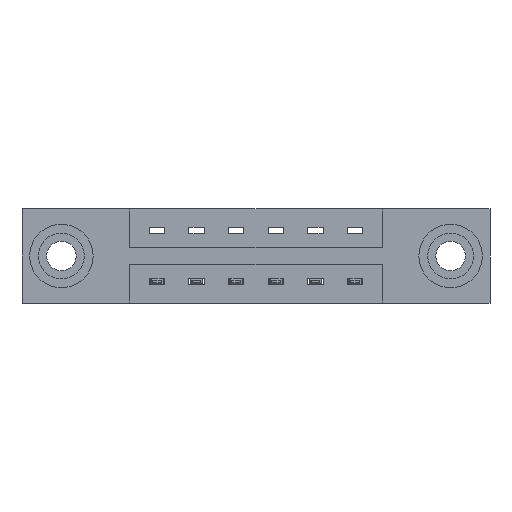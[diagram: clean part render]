
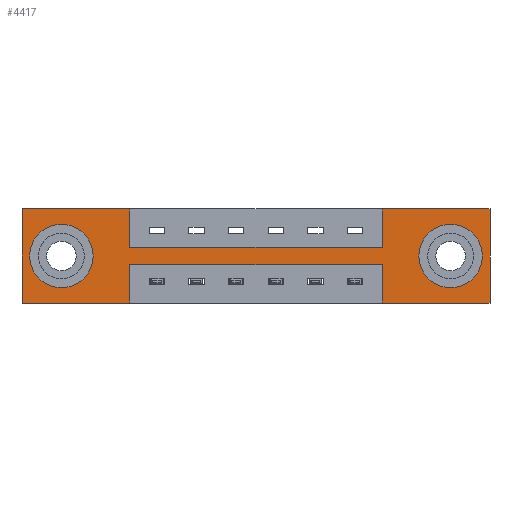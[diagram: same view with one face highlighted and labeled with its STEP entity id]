
A CAD part, front view. The second image highlights one B-rep face of the part: STEP entity #4417.
In plain terms, the highlighted planar face has unit normal (0, -1, 0).
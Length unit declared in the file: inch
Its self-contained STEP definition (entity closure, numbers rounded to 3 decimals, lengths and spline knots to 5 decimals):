
#157 = DIRECTION ( 'NONE',  ( 0., 1., 0. ) ) ;
#269 = LINE ( 'NONE', #6003, #1563 ) ;
#312 = DIRECTION ( 'NONE',  ( 0., 1., 0. ) ) ;
#375 = CARTESIAN_POINT ( 'NONE',  ( 1.842, 0., 0. ) ) ;
#409 = CARTESIAN_POINT ( 'NONE',  ( 0.155, 0., -0.185 ) ) ;
#509 = EDGE_CURVE ( 'NONE', #6867, #2785, #5692, .T. ) ;
#569 = LINE ( 'NONE', #9338, #5206 ) ;
#635 = EDGE_CURVE ( 'NONE', #3390, #4020, #8499, .T. ) ;
#655 = CARTESIAN_POINT ( 'NONE',  ( 1.842, 0., -0.37 ) ) ;
#848 = CARTESIAN_POINT ( 'NONE',  ( 0., 0., 0. ) ) ;
#894 = VERTEX_POINT ( 'NONE', #7296 ) ;
#914 = DIRECTION ( 'NONE',  ( 1., 0., 0. ) ) ;
#1069 = DIRECTION ( 'NONE',  ( 0., 1., 0. ) ) ;
#1082 = CARTESIAN_POINT ( 'NONE',  ( 0.425, 0., -0.22 ) ) ;
#1241 = LINE ( 'NONE', #4777, #5623 ) ;
#1338 = VERTEX_POINT ( 'NONE', #375 ) ;
#1384 = EDGE_CURVE ( 'NONE', #9040, #6408, #8601, .T. ) ;
#1538 = AXIS2_PLACEMENT_3D ( 'NONE', #5280, #4558, #4771 ) ;
#1563 = VECTOR ( 'NONE', #6723, 39.37008 ) ;
#1758 = VECTOR ( 'NONE', #7653, 39.37008 ) ;
#1816 = CARTESIAN_POINT ( 'NONE',  ( 0.425, 0., 0. ) ) ;
#1837 = CARTESIAN_POINT ( 'NONE',  ( 0.425, 0., 0. ) ) ;
#2112 = LINE ( 'NONE', #6411, #2921 ) ;
#2117 = DIRECTION ( 'NONE',  ( 0., 0., 1. ) ) ;
#2231 = VERTEX_POINT ( 'NONE', #6467 ) ;
#2286 = ORIENTED_EDGE ( 'NONE', *, *, #1384, .F. ) ;
#2301 = VERTEX_POINT ( 'NONE', #5776 ) ;
#2312 = ORIENTED_EDGE ( 'NONE', *, *, #6732, .F. ) ;
#2342 = LINE ( 'NONE', #9557, #4429 ) ;
#2367 = CARTESIAN_POINT ( 'NONE',  ( 1.842, 0., 0. ) ) ;
#2472 = DIRECTION ( 'NONE',  ( 0., 0., 1. ) ) ;
#2477 = VECTOR ( 'NONE', #5883, 39.37008 ) ;
#2533 = CARTESIAN_POINT ( 'NONE',  ( 0.425, 0., -0.22 ) ) ;
#2535 = DIRECTION ( 'NONE',  ( -1., 0., 0. ) ) ;
#2622 = VECTOR ( 'NONE', #4482, 39.37008 ) ;
#2672 = DIRECTION ( 'NONE',  ( 0., -1., 0. ) ) ;
#2735 = VERTEX_POINT ( 'NONE', #655 ) ;
#2780 = EDGE_CURVE ( 'NONE', #4020, #6808, #4007, .T. ) ;
#2785 = VERTEX_POINT ( 'NONE', #6301 ) ;
#2802 = EDGE_CURVE ( 'NONE', #2231, #1338, #4596, .T. ) ;
#2816 = FACE_BOUND ( 'NONE', #4846, .T. ) ;
#2878 = EDGE_CURVE ( 'NONE', #894, #3733, #4833, .T. ) ;
#2921 = VECTOR ( 'NONE', #2954, 39.37008 ) ;
#2954 = DIRECTION ( 'NONE',  ( -1., 0., 0. ) ) ;
#3221 = EDGE_LOOP ( 'NONE', ( #3447, #9387 ) ) ;
#3262 = AXIS2_PLACEMENT_3D ( 'NONE', #9319, #2672, #7879 ) ;
#3390 = VERTEX_POINT ( 'NONE', #4100 ) ;
#3436 = ORIENTED_EDGE ( 'NONE', *, *, #5127, .F. ) ;
#3447 = ORIENTED_EDGE ( 'NONE', *, *, #2878, .T. ) ;
#3528 = EDGE_CURVE ( 'NONE', #2301, #4323, #8426, .T. ) ;
#3588 = EDGE_CURVE ( 'NONE', #3733, #894, #7391, .T. ) ;
#3667 = ORIENTED_EDGE ( 'NONE', *, *, #635, .F. ) ;
#3733 = VERTEX_POINT ( 'NONE', #6242 ) ;
#3771 = EDGE_CURVE ( 'NONE', #8361, #2231, #1241, .T. ) ;
#3822 = DIRECTION ( 'NONE',  ( 0., 0., 1. ) ) ;
#3863 = CARTESIAN_POINT ( 'NONE',  ( 0., 0., -0.37 ) ) ;
#4007 = LINE ( 'NONE', #4391, #2622 ) ;
#4011 = CARTESIAN_POINT ( 'NONE',  ( 0., 0., 0. ) ) ;
#4020 = VERTEX_POINT ( 'NONE', #3863 ) ;
#4100 = CARTESIAN_POINT ( 'NONE',  ( 0.425, 0., -0.37 ) ) ;
#4121 = PLANE ( 'NONE',  #3262 ) ;
#4249 = ORIENTED_EDGE ( 'NONE', *, *, #2780, .F. ) ;
#4269 = LINE ( 'NONE', #2367, #6608 ) ;
#4323 = VERTEX_POINT ( 'NONE', #2533 ) ;
#4391 = CARTESIAN_POINT ( 'NONE',  ( 0., 0., 0. ) ) ;
#4417 = ADVANCED_FACE ( 'NONE', ( #9466, #2816, #8995 ), #4121, .T. ) ;
#4420 = ORIENTED_EDGE ( 'NONE', *, *, #7651, .T. ) ;
#4429 = VECTOR ( 'NONE', #2117, 39.37008 ) ;
#4482 = DIRECTION ( 'NONE',  ( 0., 0., 1. ) ) ;
#4558 = DIRECTION ( 'NONE',  ( 0., 1., 0. ) ) ;
#4596 = LINE ( 'NONE', #848, #9033 ) ;
#4618 = ORIENTED_EDGE ( 'NONE', *, *, #6453, .F. ) ;
#4743 = EDGE_CURVE ( 'NONE', #6408, #8361, #269, .T. ) ;
#4771 = DIRECTION ( 'NONE',  ( 0., 0., -1. ) ) ;
#4777 = CARTESIAN_POINT ( 'NONE',  ( 1.417, 0., 0. ) ) ;
#4833 = CIRCLE ( 'NONE', #1538, 0.078 ) ;
#4846 = EDGE_LOOP ( 'NONE', ( #7489, #4420 ) ) ;
#4866 = DIRECTION ( 'NONE',  ( 1., 0., 0. ) ) ;
#5127 = EDGE_CURVE ( 'NONE', #9502, #2301, #2342, .T. ) ;
#5170 = CARTESIAN_POINT ( 'NONE',  ( 0.425, 0., -0.37 ) ) ;
#5206 = VECTOR ( 'NONE', #4866, 39.37008 ) ;
#5223 = ORIENTED_EDGE ( 'NONE', *, *, #3771, .F. ) ;
#5280 = CARTESIAN_POINT ( 'NONE',  ( 1.687, 0., -0.185 ) ) ;
#5341 = CARTESIAN_POINT ( 'NONE',  ( 0., 0., -0.37 ) ) ;
#5480 = CARTESIAN_POINT ( 'NONE',  ( 1.687, 0., -0.185 ) ) ;
#5518 = DIRECTION ( 'NONE',  ( 0., 0., -1. ) ) ;
#5623 = VECTOR ( 'NONE', #2472, 39.37008 ) ;
#5692 = CIRCLE ( 'NONE', #8030, 0.078 ) ;
#5776 = CARTESIAN_POINT ( 'NONE',  ( 1.417, 0., -0.22 ) ) ;
#5789 = ORIENTED_EDGE ( 'NONE', *, *, #4743, .F. ) ;
#5883 = DIRECTION ( 'NONE',  ( 0., 0., -1. ) ) ;
#5922 = CARTESIAN_POINT ( 'NONE',  ( 0.155, 0., -0.185 ) ) ;
#6003 = CARTESIAN_POINT ( 'NONE',  ( 0.425, 0., -0.15 ) ) ;
#6229 = DIRECTION ( 'NONE',  ( 0., 0., -1. ) ) ;
#6242 = CARTESIAN_POINT ( 'NONE',  ( 1.687, 0., -0.263 ) ) ;
#6301 = CARTESIAN_POINT ( 'NONE',  ( 0.155, 0., -0.263 ) ) ;
#6408 = VERTEX_POINT ( 'NONE', #7913 ) ;
#6411 = CARTESIAN_POINT ( 'NONE',  ( 0., 0., -0.37 ) ) ;
#6453 = EDGE_CURVE ( 'NONE', #2735, #9502, #2112, .T. ) ;
#6467 = CARTESIAN_POINT ( 'NONE',  ( 1.417, 0., 0. ) ) ;
#6608 = VECTOR ( 'NONE', #5518, 39.37008 ) ;
#6723 = DIRECTION ( 'NONE',  ( 1., 0., 0. ) ) ;
#6732 = EDGE_CURVE ( 'NONE', #1338, #2735, #4269, .T. ) ;
#6793 = EDGE_LOOP ( 'NONE', ( #7401, #7076, #3436, #4618, #2312, #9042, #5223, #5789, #2286, #8994, #4249, #3667 ) ) ;
#6808 = VERTEX_POINT ( 'NONE', #4011 ) ;
#6835 = VECTOR ( 'NONE', #9435, 39.37008 ) ;
#6867 = VERTEX_POINT ( 'NONE', #7667 ) ;
#6905 = VECTOR ( 'NONE', #2535, 39.37008 ) ;
#6957 = EDGE_CURVE ( 'NONE', #6808, #9040, #569, .T. ) ;
#7076 = ORIENTED_EDGE ( 'NONE', *, *, #3528, .F. ) ;
#7296 = CARTESIAN_POINT ( 'NONE',  ( 1.687, 0., -0.107 ) ) ;
#7391 = CIRCLE ( 'NONE', #9567, 0.078 ) ;
#7401 = ORIENTED_EDGE ( 'NONE', *, *, #9405, .F. ) ;
#7489 = ORIENTED_EDGE ( 'NONE', *, *, #509, .T. ) ;
#7651 = EDGE_CURVE ( 'NONE', #2785, #6867, #7984, .T. ) ;
#7653 = DIRECTION ( 'NONE',  ( -1., 0., 0. ) ) ;
#7667 = CARTESIAN_POINT ( 'NONE',  ( 0.155, 0., -0.107 ) ) ;
#7824 = LINE ( 'NONE', #5170, #2477 ) ;
#7879 = DIRECTION ( 'NONE',  ( 0., 0., -1. ) ) ;
#7895 = CARTESIAN_POINT ( 'NONE',  ( 1.417, 0., -0.15 ) ) ;
#7913 = CARTESIAN_POINT ( 'NONE',  ( 0.425, 0., -0.15 ) ) ;
#7984 = CIRCLE ( 'NONE', #8125, 0.078 ) ;
#8030 = AXIS2_PLACEMENT_3D ( 'NONE', #5922, #157, #3822 ) ;
#8125 = AXIS2_PLACEMENT_3D ( 'NONE', #409, #312, #8457 ) ;
#8286 = CARTESIAN_POINT ( 'NONE',  ( 1.417, 0., -0.37 ) ) ;
#8361 = VERTEX_POINT ( 'NONE', #7895 ) ;
#8426 = LINE ( 'NONE', #1082, #6905 ) ;
#8457 = DIRECTION ( 'NONE',  ( 0., 0., 1. ) ) ;
#8499 = LINE ( 'NONE', #5341, #1758 ) ;
#8601 = LINE ( 'NONE', #1837, #6835 ) ;
#8994 = ORIENTED_EDGE ( 'NONE', *, *, #6957, .F. ) ;
#8995 = FACE_OUTER_BOUND ( 'NONE', #6793, .T. ) ;
#9033 = VECTOR ( 'NONE', #914, 39.37008 ) ;
#9040 = VERTEX_POINT ( 'NONE', #1816 ) ;
#9042 = ORIENTED_EDGE ( 'NONE', *, *, #2802, .F. ) ;
#9319 = CARTESIAN_POINT ( 'NONE',  ( 0., 0., -0.37 ) ) ;
#9338 = CARTESIAN_POINT ( 'NONE',  ( 0., 0., 0. ) ) ;
#9387 = ORIENTED_EDGE ( 'NONE', *, *, #3588, .T. ) ;
#9405 = EDGE_CURVE ( 'NONE', #4323, #3390, #7824, .T. ) ;
#9435 = DIRECTION ( 'NONE',  ( 0., 0., -1. ) ) ;
#9466 = FACE_BOUND ( 'NONE', #3221, .T. ) ;
#9502 = VERTEX_POINT ( 'NONE', #8286 ) ;
#9557 = CARTESIAN_POINT ( 'NONE',  ( 1.417, 0., -0.37 ) ) ;
#9567 = AXIS2_PLACEMENT_3D ( 'NONE', #5480, #1069, #6229 ) ;
